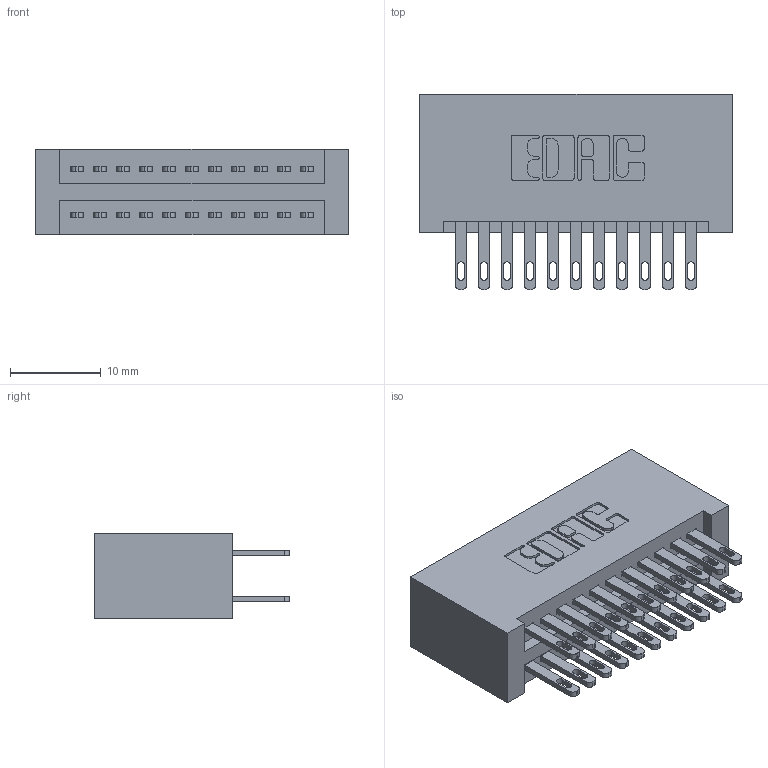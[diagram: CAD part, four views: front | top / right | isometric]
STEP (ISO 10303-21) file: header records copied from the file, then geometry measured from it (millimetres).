
FILE_DESCRIPTION (( 'STEP AP203' ), '1' );
FILE_NAME ('345-022-500-201.STEP', '2018-08-20T10:29:25', ( '' ), ( '' ), 'SwSTEP 2.0', 'SolidWorks 2016', '' );
FILE_SCHEMA (( 'CONFIG_CONTROL_DESIGN' ));
Length unit declared in the file: inch
Products named in the file (3): 345 Part_No Mounting Lugs; 345-292-001_345-293-100; 345-022-500-201
Assembly tree (23 placements, depth 2):
  345-022-500-201
    345 Part_No Mounting Lugs
    345-292-001_345-293-100  x22
Bounding box: 34.54 x 21.51 x 9.4 mm (x, y, z)
Volume: 3751 mm3; surface area: 5471.9 mm2
Topology: 23 solids, 23 shells, 1130 faces, 3419 edges, 2278 vertices
Faces by surface type: plane 670, cylinder 460
Entity records: 12457 total; most frequent: CARTESIAN_POINT 2116, ORIENTED_EDGE 2050, DIRECTION 1901, EDGE_CURVE 1025, LINE 853, VECTOR 853, VERTEX_POINT 682, AXIS2_PLACEMENT_3D 524
